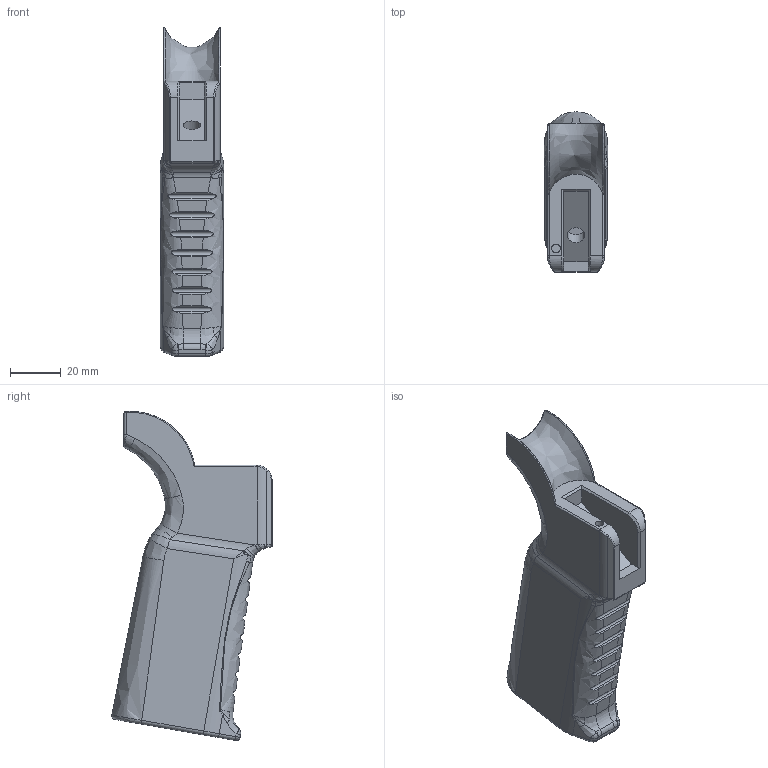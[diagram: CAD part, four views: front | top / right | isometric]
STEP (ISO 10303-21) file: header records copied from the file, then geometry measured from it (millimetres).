
FILE_DESCRIPTION(/* description */ (''),/* implementation_level */ '2;1');
FILE_NAME(/* name */ 'K Too.step',/* time_stamp */ '2021-08-15T16:35:19-04:00',/* author */ (''),/* organization */ (''),/* preprocessor_version */ 'ST-DEVELOPER v18.1',/* originating_system */ 'Autodesk Translation Framework v10.9.0.1377',/* authorisation */ '');
FILE_SCHEMA (('AUTOMOTIVE_DESIGN { 1 0 10303 214 3 1 1 }'));
Length unit declared in the file: millimetre
Products named in the file (1): K Too
Bounding box: 24.83 x 63.06 x 129.44 mm (x, y, z)
Volume: 61635.4 mm3; surface area: 26405.1 mm2
Topology: 1 solids, 1 shells, 260 faces, 627 edges, 367 vertices
Faces by surface type: bspline 112, plane 64, cylinder 57, torus 18, sphere 6, cone 3
Full cylindrical faces by diameter (mm): 3.4 x1, 6.8 x1
Entity records: 13657 total; most frequent: CARTESIAN_POINT 8451, ORIENTED_EDGE 1238, DIRECTION 791, EDGE_CURVE 619, VERTEX_POINT 367, AXIS2_PLACEMENT_3D 312, B_SPLINE_CURVE_WITH_KNOTS 289, EDGE_LOOP 268
